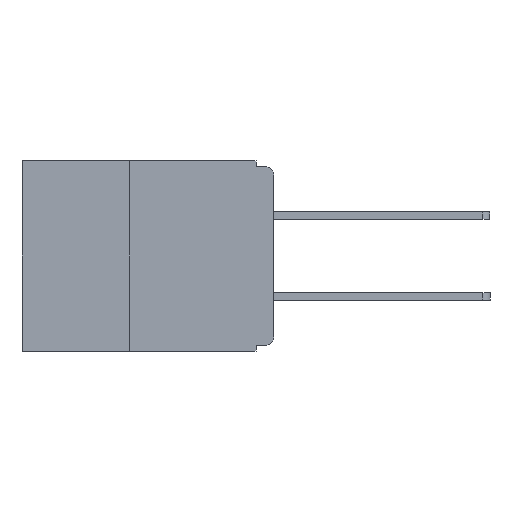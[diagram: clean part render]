
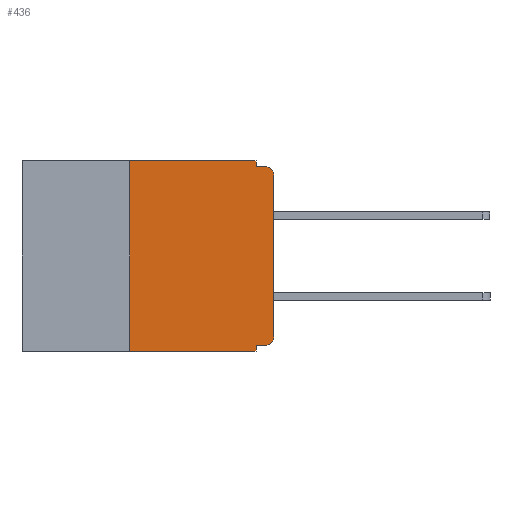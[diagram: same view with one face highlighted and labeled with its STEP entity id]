
A CAD part, left-side view. The second image highlights one B-rep face of the part: STEP entity #436.
In plain terms, the highlighted planar face has unit normal (-1, 0, 0).
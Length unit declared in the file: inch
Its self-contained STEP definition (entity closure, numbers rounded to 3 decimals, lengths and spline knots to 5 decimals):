
#186 = ORIENTED_EDGE ( 'NONE', *, *, #1958, .F. ) ;
#244 = LINE ( 'NONE', #12402, #3109 ) ;
#400 = LINE ( 'NONE', #10723, #3238 ) ;
#419 = CARTESIAN_POINT ( 'NONE',  ( 0., 0.015, -0.305 ) ) ;
#436 = ADVANCED_FACE ( 'NONE', ( #2668 ), #4837, .F. ) ;
#762 = ORIENTED_EDGE ( 'NONE', *, *, #3599, .F. ) ;
#986 = VERTEX_POINT ( 'NONE', #5692 ) ;
#1054 = CARTESIAN_POINT ( 'NONE',  ( 0., 0.015, -0.32 ) ) ;
#1473 = CARTESIAN_POINT ( 'NONE',  ( 0., 0., -0.025 ) ) ;
#1498 = DIRECTION ( 'NONE',  ( 0., 0., -1. ) ) ;
#1672 = LINE ( 'NONE', #10661, #9193 ) ;
#1718 = ORIENTED_EDGE ( 'NONE', *, *, #5126, .F. ) ;
#1958 = EDGE_CURVE ( 'NONE', #2670, #7080, #244, .T. ) ;
#2293 = VERTEX_POINT ( 'NONE', #1054 ) ;
#2334 = CARTESIAN_POINT ( 'NONE',  ( 0., 0.25, -0.33 ) ) ;
#2348 = DIRECTION ( 'NONE',  ( 0., 0., 1. ) ) ;
#2454 = DIRECTION ( 'NONE',  ( 0., 0., -1. ) ) ;
#2563 = ORIENTED_EDGE ( 'NONE', *, *, #9686, .T. ) ;
#2668 = FACE_OUTER_BOUND ( 'NONE', #7675, .T. ) ;
#2670 = VERTEX_POINT ( 'NONE', #3234 ) ;
#2959 = VERTEX_POINT ( 'NONE', #9283 ) ;
#3109 = VECTOR ( 'NONE', #2454, 39.37008 ) ;
#3153 = CARTESIAN_POINT ( 'NONE',  ( 0., 0., -0.32 ) ) ;
#3225 = VERTEX_POINT ( 'NONE', #12396 ) ;
#3234 = CARTESIAN_POINT ( 'NONE',  ( 0., 0.031, 0. ) ) ;
#3238 = VECTOR ( 'NONE', #12699, 39.37008 ) ;
#3398 = ORIENTED_EDGE ( 'NONE', *, *, #4741, .T. ) ;
#3401 = CARTESIAN_POINT ( 'NONE',  ( 0., 0., -0.305 ) ) ;
#3417 = ORIENTED_EDGE ( 'NONE', *, *, #6408, .F. ) ;
#3573 = EDGE_CURVE ( 'NONE', #5261, #3225, #8187, .T. ) ;
#3574 = CARTESIAN_POINT ( 'NONE',  ( 0., 0.437, 0. ) ) ;
#3599 = EDGE_CURVE ( 'NONE', #8989, #2670, #4854, .T. ) ;
#4000 = AXIS2_PLACEMENT_3D ( 'NONE', #419, #7696, #1498 ) ;
#4187 = DIRECTION ( 'NONE',  ( 0., 1., 0. ) ) ;
#4324 = ORIENTED_EDGE ( 'NONE', *, *, #3573, .T. ) ;
#4664 = VECTOR ( 'NONE', #5982, 39.37008 ) ;
#4741 = EDGE_CURVE ( 'NONE', #9577, #5261, #9721, .T. ) ;
#4763 = DIRECTION ( 'NONE',  ( 1., 0., 0. ) ) ;
#4837 = PLANE ( 'NONE',  #10053 ) ;
#4854 = LINE ( 'NONE', #11260, #12862 ) ;
#5126 = EDGE_CURVE ( 'NONE', #986, #8989, #10670, .T. ) ;
#5261 = VERTEX_POINT ( 'NONE', #1473 ) ;
#5327 = ORIENTED_EDGE ( 'NONE', *, *, #8716, .F. ) ;
#5671 = CARTESIAN_POINT ( 'NONE',  ( 0., 0.25, 0. ) ) ;
#5692 = CARTESIAN_POINT ( 'NONE',  ( 0., 0.25, -0.33 ) ) ;
#5773 = CARTESIAN_POINT ( 'NONE',  ( 0., 0., 0. ) ) ;
#5888 = ORIENTED_EDGE ( 'NONE', *, *, #9170, .F. ) ;
#5982 = DIRECTION ( 'NONE',  ( 0., 0., 1. ) ) ;
#6155 = VECTOR ( 'NONE', #11940, 39.37008 ) ;
#6408 = EDGE_CURVE ( 'NONE', #7808, #2959, #1672, .T. ) ;
#6448 = ORIENTED_EDGE ( 'NONE', *, *, #11779, .T. ) ;
#6474 = LINE ( 'NONE', #8896, #6155 ) ;
#7080 = VERTEX_POINT ( 'NONE', #8681 ) ;
#7410 = LINE ( 'NONE', #3153, #9107 ) ;
#7532 = DIRECTION ( 'NONE',  ( 0., 0., -1. ) ) ;
#7675 = EDGE_LOOP ( 'NONE', ( #3398, #4324, #5888, #186, #762, #1718, #2563, #3417, #5327, #6448 ) ) ;
#7696 = DIRECTION ( 'NONE',  ( -1., 0., 0. ) ) ;
#7808 = VERTEX_POINT ( 'NONE', #8828 ) ;
#8187 = CIRCLE ( 'NONE', #10678, 0.015 ) ;
#8292 = VECTOR ( 'NONE', #2348, 39.37008 ) ;
#8681 = CARTESIAN_POINT ( 'NONE',  ( 0., 0.031, -0.01 ) ) ;
#8716 = EDGE_CURVE ( 'NONE', #2293, #7808, #7410, .T. ) ;
#8828 = CARTESIAN_POINT ( 'NONE',  ( 0., 0.031, -0.32 ) ) ;
#8896 = CARTESIAN_POINT ( 'NONE',  ( 0., 0., -0.01 ) ) ;
#8989 = VERTEX_POINT ( 'NONE', #5671 ) ;
#9107 = VECTOR ( 'NONE', #4187, 39.37008 ) ;
#9170 = EDGE_CURVE ( 'NONE', #7080, #3225, #6474, .T. ) ;
#9193 = VECTOR ( 'NONE', #9629, 39.37008 ) ;
#9283 = CARTESIAN_POINT ( 'NONE',  ( 0., 0.031, -0.33 ) ) ;
#9577 = VERTEX_POINT ( 'NONE', #3401 ) ;
#9629 = DIRECTION ( 'NONE',  ( 0., 0., -1. ) ) ;
#9686 = EDGE_CURVE ( 'NONE', #986, #2959, #400, .T. ) ;
#9721 = LINE ( 'NONE', #5773, #4664 ) ;
#10053 = AXIS2_PLACEMENT_3D ( 'NONE', #3574, #4763, #7532 ) ;
#10661 = CARTESIAN_POINT ( 'NONE',  ( 0., 0.031, -0.33 ) ) ;
#10670 = LINE ( 'NONE', #2334, #8292 ) ;
#10678 = AXIS2_PLACEMENT_3D ( 'NONE', #12333, #12304, #11747 ) ;
#10723 = CARTESIAN_POINT ( 'NONE',  ( 0., 0.437, -0.33 ) ) ;
#11177 = DIRECTION ( 'NONE',  ( 0., -1., 0. ) ) ;
#11260 = CARTESIAN_POINT ( 'NONE',  ( 0., 0.437, 0. ) ) ;
#11747 = DIRECTION ( 'NONE',  ( 0., 0., -1. ) ) ;
#11779 = EDGE_CURVE ( 'NONE', #2293, #9577, #11893, .T. ) ;
#11893 = CIRCLE ( 'NONE', #4000, 0.015 ) ;
#11940 = DIRECTION ( 'NONE',  ( 0., -1., 0. ) ) ;
#12304 = DIRECTION ( 'NONE',  ( -1., 0., 0. ) ) ;
#12333 = CARTESIAN_POINT ( 'NONE',  ( 0., 0.015, -0.025 ) ) ;
#12396 = CARTESIAN_POINT ( 'NONE',  ( 0., 0.015, -0.01 ) ) ;
#12402 = CARTESIAN_POINT ( 'NONE',  ( 0., 0.031, 0. ) ) ;
#12699 = DIRECTION ( 'NONE',  ( 0., -1., 0. ) ) ;
#12862 = VECTOR ( 'NONE', #11177, 39.37008 ) ;
